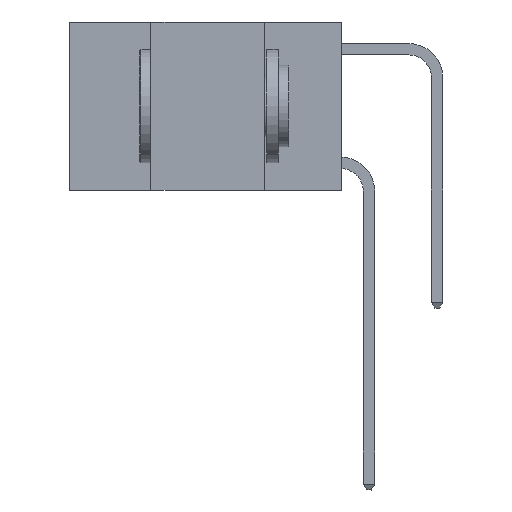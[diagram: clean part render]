
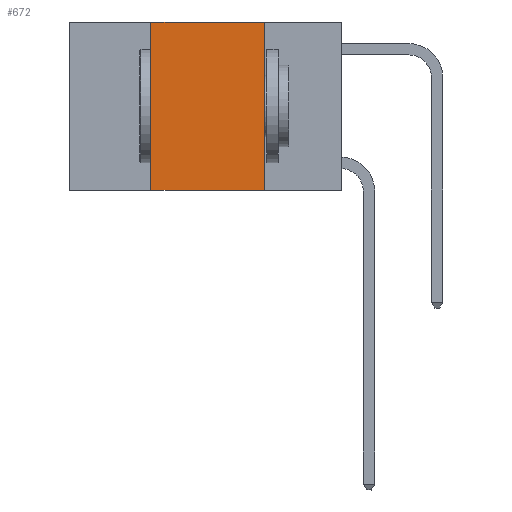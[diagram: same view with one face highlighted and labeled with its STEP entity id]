
A CAD part, left-side view. The second image highlights one B-rep face of the part: STEP entity #672.
In plain terms, the highlighted planar face has unit normal (-1, 0, 0).
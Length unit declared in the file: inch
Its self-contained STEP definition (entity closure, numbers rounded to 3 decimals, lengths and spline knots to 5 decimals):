
#349 = EDGE_CURVE ( 'NONE', #2697, #1345, #4712, .T. ) ;
#452 = ORIENTED_EDGE ( 'NONE', *, *, #349, .F. ) ;
#515 = DIRECTION ( 'NONE',  ( 0., -1., 0. ) ) ;
#672 = ADVANCED_FACE ( 'NONE', ( #11270 ), #8796, .F. ) ;
#1210 = VECTOR ( 'NONE', #10482, 39.37008 ) ;
#1345 = VERTEX_POINT ( 'NONE', #5465 ) ;
#2697 = VERTEX_POINT ( 'NONE', #5346 ) ;
#2813 = CARTESIAN_POINT ( 'NONE',  ( 0., 0.17, -0.37 ) ) ;
#3273 = VERTEX_POINT ( 'NONE', #2813 ) ;
#3357 = DIRECTION ( 'NONE',  ( 0., 0., -1. ) ) ;
#3827 = VECTOR ( 'NONE', #515, 39.37008 ) ;
#4125 = VECTOR ( 'NONE', #9583, 39.37008 ) ;
#4168 = DIRECTION ( 'NONE',  ( 0., 0., -1. ) ) ;
#4712 = LINE ( 'NONE', #10473, #4125 ) ;
#4873 = AXIS2_PLACEMENT_3D ( 'NONE', #7713, #7132, #3357 ) ;
#5160 = EDGE_CURVE ( 'NONE', #2697, #3273, #6110, .T. ) ;
#5346 = CARTESIAN_POINT ( 'NONE',  ( 0., 0.42, -0.37 ) ) ;
#5465 = CARTESIAN_POINT ( 'NONE',  ( 0., 0.42, 0. ) ) ;
#5540 = LINE ( 'NONE', #5917, #6680 ) ;
#5573 = CARTESIAN_POINT ( 'NONE',  ( 0., 0.17, 0. ) ) ;
#5917 = CARTESIAN_POINT ( 'NONE',  ( 0., 0.17, 0. ) ) ;
#6110 = LINE ( 'NONE', #10486, #3827 ) ;
#6680 = VECTOR ( 'NONE', #4168, 39.37008 ) ;
#7132 = DIRECTION ( 'NONE',  ( 1., 0., 0. ) ) ;
#7713 = CARTESIAN_POINT ( 'NONE',  ( 0., 0.6, 0. ) ) ;
#8615 = EDGE_LOOP ( 'NONE', ( #8643, #11446, #452, #10030 ) ) ;
#8643 = ORIENTED_EDGE ( 'NONE', *, *, #9076, .F. ) ;
#8796 = PLANE ( 'NONE',  #4873 ) ;
#8825 = LINE ( 'NONE', #10411, #1210 ) ;
#9076 = EDGE_CURVE ( 'NONE', #10289, #3273, #5540, .T. ) ;
#9339 = EDGE_CURVE ( 'NONE', #1345, #10289, #8825, .T. ) ;
#9583 = DIRECTION ( 'NONE',  ( 0., 0., 1. ) ) ;
#10030 = ORIENTED_EDGE ( 'NONE', *, *, #5160, .T. ) ;
#10289 = VERTEX_POINT ( 'NONE', #5573 ) ;
#10411 = CARTESIAN_POINT ( 'NONE',  ( 0., 0.6, 0. ) ) ;
#10473 = CARTESIAN_POINT ( 'NONE',  ( 0., 0.42, 0. ) ) ;
#10482 = DIRECTION ( 'NONE',  ( 0., -1., 0. ) ) ;
#10486 = CARTESIAN_POINT ( 'NONE',  ( 0., 0.6, -0.37 ) ) ;
#11270 = FACE_OUTER_BOUND ( 'NONE', #8615, .T. ) ;
#11446 = ORIENTED_EDGE ( 'NONE', *, *, #9339, .F. ) ;
